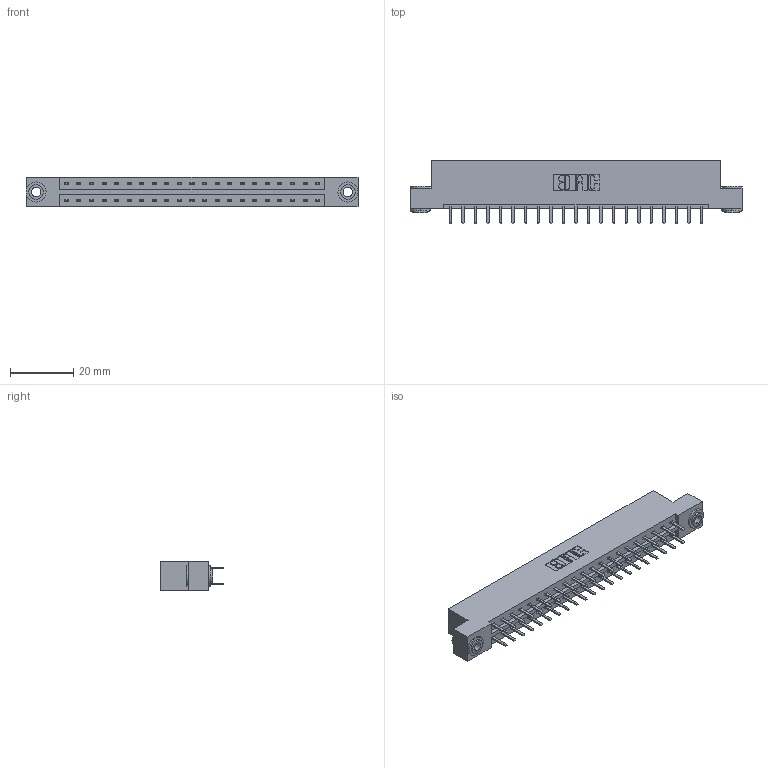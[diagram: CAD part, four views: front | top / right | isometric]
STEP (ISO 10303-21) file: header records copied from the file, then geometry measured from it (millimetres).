
FILE_DESCRIPTION (( 'STEP AP203' ), '1' );
FILE_NAME ('833-042-520-203.STEP', '2020-06-03T20:12:28', ( '' ), ( '' ), 'SwSTEP 2.0', 'SolidWorks 2020', '' );
FILE_SCHEMA (( 'CONFIG_CONTROL_DESIGN' ));
Length unit declared in the file: inch
Products named in the file (4): 345-250-002_345-250-002-102; 345-292-001_345-293-120; 833-042-520-203; 833 Part_Flush - .156 Dia - TH
Assembly tree (45 placements, depth 2):
  833-042-520-203
    833 Part_Flush - .156 Dia - TH
    345-292-001_345-293-120  x42
    345-250-002_345-250-002-102  x2
Bounding box: 104.75 x 20.02 x 9.4 mm (x, y, z)
Volume: 10498.9 mm3; surface area: 12358.6 mm2
Topology: 45 solids, 45 shells, 2504 faces, 7233 edges, 4706 vertices
Faces by surface type: plane 1676, cylinder 820, cone 8
Entity records: 16990 total; most frequent: CARTESIAN_POINT 2829, ORIENTED_EDGE 2746, DIRECTION 2475, EDGE_CURVE 1373, VECTOR 1217, LINE 1217, VERTEX_POINT 910, AXIS2_PLACEMENT_3D 629
